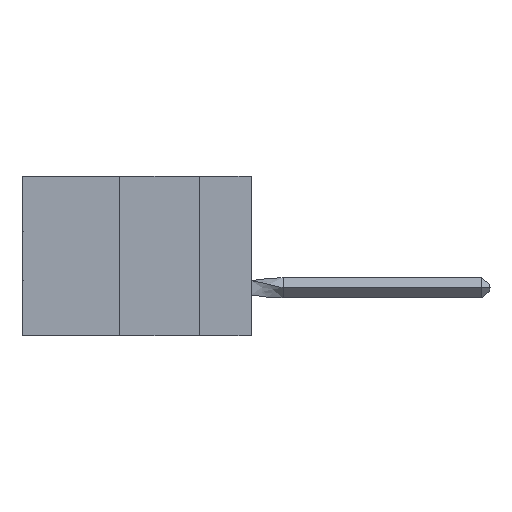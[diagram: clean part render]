
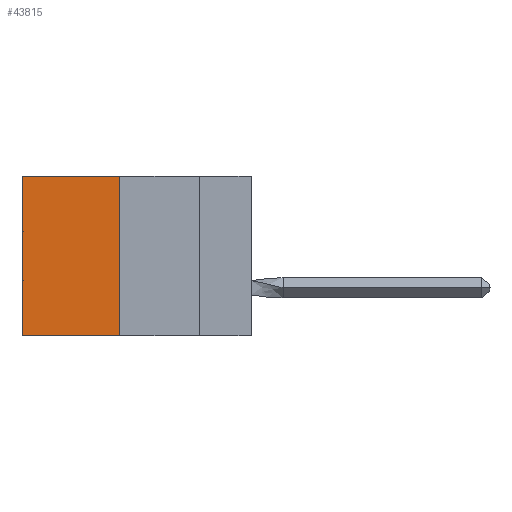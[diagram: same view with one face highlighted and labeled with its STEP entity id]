
A CAD part, left-side view. The second image highlights one B-rep face of the part: STEP entity #43815.
In plain terms, the highlighted planar face has unit normal (-1, 0, 0).
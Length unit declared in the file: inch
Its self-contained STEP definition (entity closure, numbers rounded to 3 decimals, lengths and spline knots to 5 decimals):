
#1837 = DIRECTION ( 'NONE',  ( 0., 1., 0. ) ) ;
#2627 = ORIENTED_EDGE ( 'NONE', *, *, #30253, .F. ) ;
#3868 = DIRECTION ( 'NONE',  ( 0., 0., -1. ) ) ;
#5201 = CARTESIAN_POINT ( 'NONE',  ( 0.305, 0.413, -0.5 ) ) ;
#5355 = DIRECTION ( 'NONE',  ( 0., 0., -1. ) ) ;
#6049 = VECTOR ( 'NONE', #5355, 39.37008 ) ;
#7645 = VECTOR ( 'NONE', #34905, 39.37008 ) ;
#11145 = VERTEX_POINT ( 'NONE', #37053 ) ;
#13681 = CARTESIAN_POINT ( 'NONE',  ( 0.305, 0.413, 0. ) ) ;
#14198 = VERTEX_POINT ( 'NONE', #17053 ) ;
#14369 = LINE ( 'NONE', #34839, #22559 ) ;
#14450 = PLANE ( 'NONE',  #20801 ) ;
#15608 = VECTOR ( 'NONE', #1837, 39.37008 ) ;
#17053 = CARTESIAN_POINT ( 'NONE',  ( 0.305, 0.72, -0.5 ) ) ;
#17192 = DIRECTION ( 'NONE',  ( 0., 0., -1. ) ) ;
#18144 = DIRECTION ( 'NONE',  ( 1., 0., 0. ) ) ;
#18296 = ORIENTED_EDGE ( 'NONE', *, *, #33912, .T. ) ;
#18507 = VERTEX_POINT ( 'NONE', #34886 ) ;
#20801 = AXIS2_PLACEMENT_3D ( 'NONE', #39195, #18144, #3868 ) ;
#22559 = VECTOR ( 'NONE', #17192, 39.37008 ) ;
#23154 = CARTESIAN_POINT ( 'NONE',  ( 0.305, 0.413, -0.5 ) ) ;
#25083 = ORIENTED_EDGE ( 'NONE', *, *, #29557, .T. ) ;
#27935 = VERTEX_POINT ( 'NONE', #36016 ) ;
#29557 = EDGE_CURVE ( 'NONE', #27935, #14198, #14369, .T. ) ;
#30253 = EDGE_CURVE ( 'NONE', #18507, #11145, #35181, .T. ) ;
#33912 = EDGE_CURVE ( 'NONE', #18507, #27935, #42854, .T. ) ;
#34839 = CARTESIAN_POINT ( 'NONE',  ( 0.305, 0.72, -0.5 ) ) ;
#34886 = CARTESIAN_POINT ( 'NONE',  ( 0.305, 0.413, 0. ) ) ;
#34905 = DIRECTION ( 'NONE',  ( 0., 1., 0. ) ) ;
#35181 = LINE ( 'NONE', #5201, #6049 ) ;
#36016 = CARTESIAN_POINT ( 'NONE',  ( 0.305, 0.72, 0. ) ) ;
#37053 = CARTESIAN_POINT ( 'NONE',  ( 0.305, 0.413, -0.5 ) ) ;
#39195 = CARTESIAN_POINT ( 'NONE',  ( 0.305, 0.413, -0.5 ) ) ;
#39200 = ORIENTED_EDGE ( 'NONE', *, *, #39246, .F. ) ;
#39226 = LINE ( 'NONE', #23154, #15608 ) ;
#39246 = EDGE_CURVE ( 'NONE', #11145, #14198, #39226, .T. ) ;
#41856 = EDGE_LOOP ( 'NONE', ( #25083, #39200, #2627, #18296 ) ) ;
#42660 = FACE_OUTER_BOUND ( 'NONE', #41856, .T. ) ;
#42854 = LINE ( 'NONE', #13681, #7645 ) ;
#43815 = ADVANCED_FACE ( 'NONE', ( #42660 ), #14450, .F. ) ;
